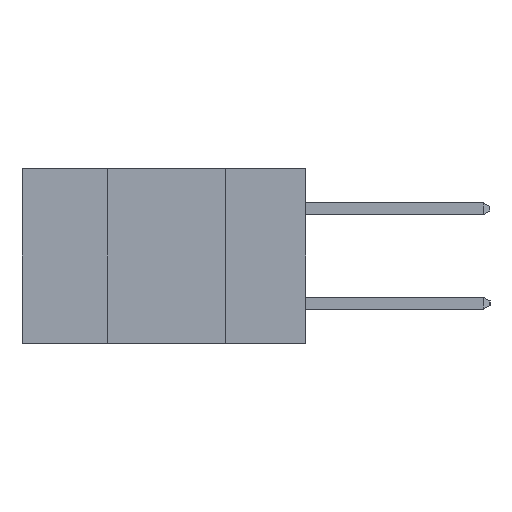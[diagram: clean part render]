
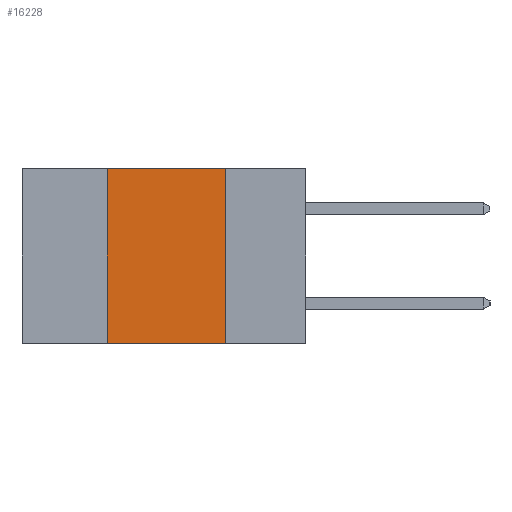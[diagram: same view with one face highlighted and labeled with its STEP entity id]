
A CAD part, left-side view. The second image highlights one B-rep face of the part: STEP entity #16228.
In plain terms, the highlighted planar face has unit normal (-1, 0, 0).
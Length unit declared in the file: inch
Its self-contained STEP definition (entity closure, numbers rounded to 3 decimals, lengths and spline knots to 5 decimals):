
#461 = VECTOR ( 'NONE', #5143, 39.37008 ) ;
#1888 = EDGE_CURVE ( 'NONE', #10770, #10171, #6208, .T. ) ;
#2670 = VECTOR ( 'NONE', #11732, 39.37008 ) ;
#4569 = CARTESIAN_POINT ( 'NONE',  ( 0., 0.42, -0.37 ) ) ;
#5143 = DIRECTION ( 'NONE',  ( 0., 0., 1. ) ) ;
#5585 = CARTESIAN_POINT ( 'NONE',  ( 0., 0.17, 0. ) ) ;
#5743 = CARTESIAN_POINT ( 'NONE',  ( 0., 0.17, -0.37 ) ) ;
#6208 = LINE ( 'NONE', #24079, #461 ) ;
#7433 = CARTESIAN_POINT ( 'NONE',  ( 0., 0.6, 0. ) ) ;
#7849 = CARTESIAN_POINT ( 'NONE',  ( 0., 0.6, -0.37 ) ) ;
#8471 = VERTEX_POINT ( 'NONE', #5585 ) ;
#9612 = EDGE_CURVE ( 'NONE', #10171, #8471, #14068, .T. ) ;
#10171 = VERTEX_POINT ( 'NONE', #21896 ) ;
#10602 = ORIENTED_EDGE ( 'NONE', *, *, #26592, .T. ) ;
#10686 = ORIENTED_EDGE ( 'NONE', *, *, #1888, .F. ) ;
#10770 = VERTEX_POINT ( 'NONE', #4569 ) ;
#11699 = ORIENTED_EDGE ( 'NONE', *, *, #9612, .F. ) ;
#11732 = DIRECTION ( 'NONE',  ( 0., -1., 0. ) ) ;
#12126 = CARTESIAN_POINT ( 'NONE',  ( 0., 0.6, 0. ) ) ;
#12223 = DIRECTION ( 'NONE',  ( 1., 0., 0. ) ) ;
#13182 = VECTOR ( 'NONE', #18356, 39.37008 ) ;
#13787 = ORIENTED_EDGE ( 'NONE', *, *, #16931, .F. ) ;
#14068 = LINE ( 'NONE', #7433, #2670 ) ;
#14510 = LINE ( 'NONE', #7849, #13182 ) ;
#15596 = AXIS2_PLACEMENT_3D ( 'NONE', #12126, #12223, #26778 ) ;
#15780 = FACE_OUTER_BOUND ( 'NONE', #16479, .T. ) ;
#16228 = ADVANCED_FACE ( 'NONE', ( #15780 ), #24715, .F. ) ;
#16479 = EDGE_LOOP ( 'NONE', ( #13787, #11699, #10686, #10602 ) ) ;
#16931 = EDGE_CURVE ( 'NONE', #8471, #25399, #21611, .T. ) ;
#18356 = DIRECTION ( 'NONE',  ( 0., -1., 0. ) ) ;
#19032 = DIRECTION ( 'NONE',  ( 0., 0., -1. ) ) ;
#21611 = LINE ( 'NONE', #25207, #26465 ) ;
#21896 = CARTESIAN_POINT ( 'NONE',  ( 0., 0.42, 0. ) ) ;
#24079 = CARTESIAN_POINT ( 'NONE',  ( 0., 0.42, -0.37 ) ) ;
#24715 = PLANE ( 'NONE',  #15596 ) ;
#25207 = CARTESIAN_POINT ( 'NONE',  ( 0., 0.17, -0.37 ) ) ;
#25399 = VERTEX_POINT ( 'NONE', #5743 ) ;
#26465 = VECTOR ( 'NONE', #19032, 39.37008 ) ;
#26592 = EDGE_CURVE ( 'NONE', #10770, #25399, #14510, .T. ) ;
#26778 = DIRECTION ( 'NONE',  ( 0., 0., -1. ) ) ;
